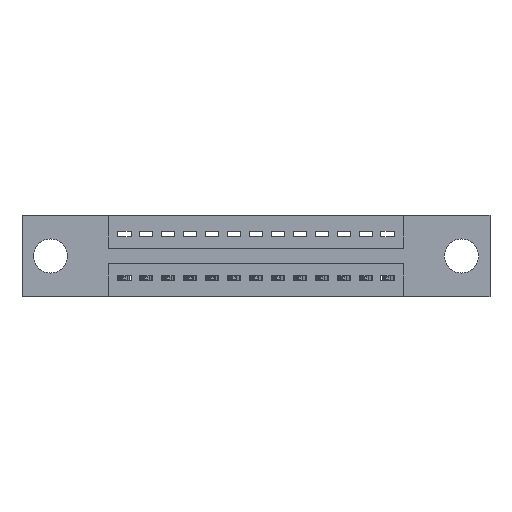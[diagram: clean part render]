
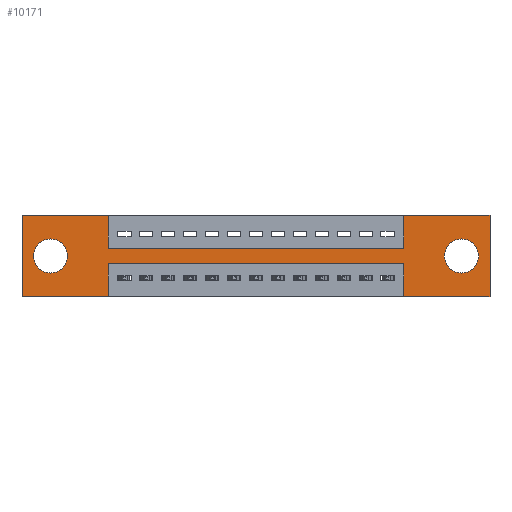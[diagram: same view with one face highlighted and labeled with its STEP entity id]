
A CAD part, front view. The second image highlights one B-rep face of the part: STEP entity #10171.
In plain terms, the highlighted planar face has unit normal (0, -1, 0).
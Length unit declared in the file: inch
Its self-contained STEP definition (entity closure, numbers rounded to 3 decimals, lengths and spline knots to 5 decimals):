
#20 = ORIENTED_EDGE ( 'NONE', *, *, #8000, .F. ) ;
#23 = CARTESIAN_POINT ( 'NONE',  ( 0.13, 0., -0.185 ) ) ;
#169 = ORIENTED_EDGE ( 'NONE', *, *, #12257, .F. ) ;
#256 = EDGE_CURVE ( 'NONE', #1904, #11613, #899, .T. ) ;
#381 = ORIENTED_EDGE ( 'NONE', *, *, #7747, .F. ) ;
#418 = ORIENTED_EDGE ( 'NONE', *, *, #8654, .F. ) ;
#558 = LINE ( 'NONE', #4926, #13770 ) ;
#782 = EDGE_CURVE ( 'NONE', #5217, #11632, #12013, .T. ) ;
#826 = DIRECTION ( 'NONE',  ( 0., 0., 1. ) ) ;
#899 = LINE ( 'NONE', #11713, #10236 ) ;
#1327 = DIRECTION ( 'NONE',  ( 0., 1., 0. ) ) ;
#1783 = DIRECTION ( 'NONE',  ( 1., 0., 0. ) ) ;
#1797 = DIRECTION ( 'NONE',  ( 0., -1., 0. ) ) ;
#1904 = VERTEX_POINT ( 'NONE', #13633 ) ;
#1942 = DIRECTION ( 'NONE',  ( 0., 0., -1. ) ) ;
#2031 = LINE ( 'NONE', #2975, #2146 ) ;
#2079 = FACE_OUTER_BOUND ( 'NONE', #4167, .T. ) ;
#2141 = CARTESIAN_POINT ( 'NONE',  ( 0.3925, 0., -0.22 ) ) ;
#2146 = VECTOR ( 'NONE', #4105, 39.37008 ) ;
#2236 = ORIENTED_EDGE ( 'NONE', *, *, #11254, .F. ) ;
#2309 = VERTEX_POINT ( 'NONE', #9805 ) ;
#2464 = CARTESIAN_POINT ( 'NONE',  ( 2.135, 0., -0.37 ) ) ;
#2683 = VERTEX_POINT ( 'NONE', #9140 ) ;
#2729 = EDGE_CURVE ( 'NONE', #2683, #10376, #6067, .T. ) ;
#2782 = ORIENTED_EDGE ( 'NONE', *, *, #12958, .T. ) ;
#2831 = VECTOR ( 'NONE', #10057, 39.37008 ) ;
#2916 = LINE ( 'NONE', #12854, #11958 ) ;
#2946 = PLANE ( 'NONE',  #7078 ) ;
#2975 = CARTESIAN_POINT ( 'NONE',  ( 0.3925, 0., -0.22 ) ) ;
#3383 = ORIENTED_EDGE ( 'NONE', *, *, #256, .F. ) ;
#3384 = DIRECTION ( 'NONE',  ( 0., 0., 1. ) ) ;
#3388 = CARTESIAN_POINT ( 'NONE',  ( 1.7425, 0., 0. ) ) ;
#3453 = DIRECTION ( 'NONE',  ( 1., 0., 0. ) ) ;
#3736 = VERTEX_POINT ( 'NONE', #4512 ) ;
#3911 = CARTESIAN_POINT ( 'NONE',  ( 0.13, 0., -0.107 ) ) ;
#3921 = CARTESIAN_POINT ( 'NONE',  ( 0., 0., 0. ) ) ;
#3927 = ORIENTED_EDGE ( 'NONE', *, *, #8580, .T. ) ;
#3935 = VERTEX_POINT ( 'NONE', #4998 ) ;
#3997 = CARTESIAN_POINT ( 'NONE',  ( 1.7425, 0., -0.22 ) ) ;
#4105 = DIRECTION ( 'NONE',  ( -1., 0., 0. ) ) ;
#4106 = CARTESIAN_POINT ( 'NONE',  ( 2.005, 0., -0.185 ) ) ;
#4150 = FACE_BOUND ( 'NONE', #10362, .T. ) ;
#4167 = EDGE_LOOP ( 'NONE', ( #13440, #20, #381, #2236, #3383, #418, #8805, #13318, #11495, #8128, #9824, #169 ) ) ;
#4265 = VERTEX_POINT ( 'NONE', #2141 ) ;
#4358 = AXIS2_PLACEMENT_3D ( 'NONE', #23, #4599, #3384 ) ;
#4459 = LINE ( 'NONE', #5598, #11380 ) ;
#4512 = CARTESIAN_POINT ( 'NONE',  ( 1.7425, 0., -0.37 ) ) ;
#4599 = DIRECTION ( 'NONE',  ( 0., 1., 0. ) ) ;
#4708 = LINE ( 'NONE', #5487, #2831 ) ;
#4787 = VECTOR ( 'NONE', #11643, 39.37008 ) ;
#4926 = CARTESIAN_POINT ( 'NONE',  ( 1.7425, 0., 0. ) ) ;
#4966 = CARTESIAN_POINT ( 'NONE',  ( 0.3925, 0., 0. ) ) ;
#4993 = DIRECTION ( 'NONE',  ( 0., 0., 1. ) ) ;
#4998 = CARTESIAN_POINT ( 'NONE',  ( 0., 0., -0.37 ) ) ;
#5043 = VERTEX_POINT ( 'NONE', #3388 ) ;
#5054 = LINE ( 'NONE', #13845, #12786 ) ;
#5217 = VERTEX_POINT ( 'NONE', #9961 ) ;
#5415 = CARTESIAN_POINT ( 'NONE',  ( 0.3925, 0., -0.37 ) ) ;
#5487 = CARTESIAN_POINT ( 'NONE',  ( 1.7425, 0., -0.37 ) ) ;
#5597 = ORIENTED_EDGE ( 'NONE', *, *, #12133, .T. ) ;
#5598 = CARTESIAN_POINT ( 'NONE',  ( 0., 0., 0. ) ) ;
#5693 = VERTEX_POINT ( 'NONE', #3911 ) ;
#5786 = EDGE_CURVE ( 'NONE', #3935, #2683, #2916, .T. ) ;
#5888 = EDGE_LOOP ( 'NONE', ( #2782, #11928 ) ) ;
#6067 = LINE ( 'NONE', #3921, #7839 ) ;
#6074 = CARTESIAN_POINT ( 'NONE',  ( 0.3925, 0., -0.15 ) ) ;
#6271 = DIRECTION ( 'NONE',  ( 1., 0., 0. ) ) ;
#6428 = CARTESIAN_POINT ( 'NONE',  ( 0., 0., -0.37 ) ) ;
#7078 = AXIS2_PLACEMENT_3D ( 'NONE', #6428, #1797, #1942 ) ;
#7083 = DIRECTION ( 'NONE',  ( 0., 1., 0. ) ) ;
#7095 = AXIS2_PLACEMENT_3D ( 'NONE', #8164, #1327, #13897 ) ;
#7261 = DIRECTION ( 'NONE',  ( 0., 0., -1. ) ) ;
#7472 = EDGE_CURVE ( 'NONE', #12076, #5043, #558, .T. ) ;
#7664 = CARTESIAN_POINT ( 'NONE',  ( 0.13, 0., -0.263 ) ) ;
#7690 = VERTEX_POINT ( 'NONE', #11992 ) ;
#7747 = EDGE_CURVE ( 'NONE', #3736, #10830, #4708, .T. ) ;
#7774 = CIRCLE ( 'NONE', #4358, 0.078 ) ;
#7783 = VECTOR ( 'NONE', #9770, 39.37008 ) ;
#7839 = VECTOR ( 'NONE', #6271, 39.37008 ) ;
#7993 = VECTOR ( 'NONE', #9660, 39.37008 ) ;
#8000 = EDGE_CURVE ( 'NONE', #10830, #4265, #2031, .T. ) ;
#8128 = ORIENTED_EDGE ( 'NONE', *, *, #2729, .F. ) ;
#8164 = CARTESIAN_POINT ( 'NONE',  ( 2.005, 0., -0.185 ) ) ;
#8275 = LINE ( 'NONE', #9642, #4787 ) ;
#8363 = CARTESIAN_POINT ( 'NONE',  ( 1.7425, 0., -0.15 ) ) ;
#8457 = DIRECTION ( 'NONE',  ( 0., 1., 0. ) ) ;
#8580 = EDGE_CURVE ( 'NONE', #8603, #5693, #7774, .T. ) ;
#8581 = AXIS2_PLACEMENT_3D ( 'NONE', #4106, #8457, #12847 ) ;
#8603 = VERTEX_POINT ( 'NONE', #7664 ) ;
#8654 = EDGE_CURVE ( 'NONE', #5043, #1904, #4459, .T. ) ;
#8805 = ORIENTED_EDGE ( 'NONE', *, *, #7472, .F. ) ;
#8917 = AXIS2_PLACEMENT_3D ( 'NONE', #11388, #7083, #10520 ) ;
#9140 = CARTESIAN_POINT ( 'NONE',  ( 0., 0., 0. ) ) ;
#9486 = DIRECTION ( 'NONE',  ( -1., 0., 0. ) ) ;
#9642 = CARTESIAN_POINT ( 'NONE',  ( 0.3925, 0., 0. ) ) ;
#9660 = DIRECTION ( 'NONE',  ( -1., 0., 0. ) ) ;
#9770 = DIRECTION ( 'NONE',  ( 0., 0., -1. ) ) ;
#9805 = CARTESIAN_POINT ( 'NONE',  ( 0.3925, 0., -0.15 ) ) ;
#9824 = ORIENTED_EDGE ( 'NONE', *, *, #5786, .F. ) ;
#9876 = LINE ( 'NONE', #11805, #7993 ) ;
#9961 = CARTESIAN_POINT ( 'NONE',  ( 2.005, 0., -0.263 ) ) ;
#10045 = CARTESIAN_POINT ( 'NONE',  ( 2.005, 0., -0.107 ) ) ;
#10057 = DIRECTION ( 'NONE',  ( 0., 0., 1. ) ) ;
#10171 = ADVANCED_FACE ( 'NONE', ( #11737, #4150, #2079 ), #2946, .T. ) ;
#10236 = VECTOR ( 'NONE', #7261, 39.37008 ) ;
#10362 = EDGE_LOOP ( 'NONE', ( #5597, #3927 ) ) ;
#10376 = VERTEX_POINT ( 'NONE', #4966 ) ;
#10520 = DIRECTION ( 'NONE',  ( 0., 0., 1. ) ) ;
#10830 = VERTEX_POINT ( 'NONE', #3997 ) ;
#10846 = LINE ( 'NONE', #5415, #7783 ) ;
#10853 = EDGE_CURVE ( 'NONE', #2309, #12076, #13722, .T. ) ;
#10896 = EDGE_CURVE ( 'NONE', #10376, #2309, #8275, .T. ) ;
#10984 = CIRCLE ( 'NONE', #7095, 0.078 ) ;
#11254 = EDGE_CURVE ( 'NONE', #11613, #3736, #5054, .T. ) ;
#11380 = VECTOR ( 'NONE', #3453, 39.37008 ) ;
#11388 = CARTESIAN_POINT ( 'NONE',  ( 0.13, 0., -0.185 ) ) ;
#11495 = ORIENTED_EDGE ( 'NONE', *, *, #10896, .F. ) ;
#11613 = VERTEX_POINT ( 'NONE', #2464 ) ;
#11632 = VERTEX_POINT ( 'NONE', #10045 ) ;
#11643 = DIRECTION ( 'NONE',  ( 0., 0., -1. ) ) ;
#11713 = CARTESIAN_POINT ( 'NONE',  ( 2.135, 0., 0. ) ) ;
#11737 = FACE_BOUND ( 'NONE', #5888, .T. ) ;
#11805 = CARTESIAN_POINT ( 'NONE',  ( 0., 0., -0.37 ) ) ;
#11889 = CIRCLE ( 'NONE', #8917, 0.078 ) ;
#11928 = ORIENTED_EDGE ( 'NONE', *, *, #782, .T. ) ;
#11958 = VECTOR ( 'NONE', #826, 39.37008 ) ;
#11992 = CARTESIAN_POINT ( 'NONE',  ( 0.3925, 0., -0.37 ) ) ;
#12013 = CIRCLE ( 'NONE', #8581, 0.078 ) ;
#12076 = VERTEX_POINT ( 'NONE', #8363 ) ;
#12133 = EDGE_CURVE ( 'NONE', #5693, #8603, #11889, .T. ) ;
#12257 = EDGE_CURVE ( 'NONE', #7690, #3935, #9876, .T. ) ;
#12774 = EDGE_CURVE ( 'NONE', #4265, #7690, #10846, .T. ) ;
#12786 = VECTOR ( 'NONE', #9486, 39.37008 ) ;
#12847 = DIRECTION ( 'NONE',  ( 0., 0., -1. ) ) ;
#12854 = CARTESIAN_POINT ( 'NONE',  ( 0., 0., 0. ) ) ;
#12958 = EDGE_CURVE ( 'NONE', #11632, #5217, #10984, .T. ) ;
#13318 = ORIENTED_EDGE ( 'NONE', *, *, #10853, .F. ) ;
#13440 = ORIENTED_EDGE ( 'NONE', *, *, #12774, .F. ) ;
#13465 = VECTOR ( 'NONE', #1783, 39.37008 ) ;
#13633 = CARTESIAN_POINT ( 'NONE',  ( 2.135, 0., 0. ) ) ;
#13722 = LINE ( 'NONE', #6074, #13465 ) ;
#13770 = VECTOR ( 'NONE', #4993, 39.37008 ) ;
#13845 = CARTESIAN_POINT ( 'NONE',  ( 0., 0., -0.37 ) ) ;
#13897 = DIRECTION ( 'NONE',  ( 0., 0., -1. ) ) ;
